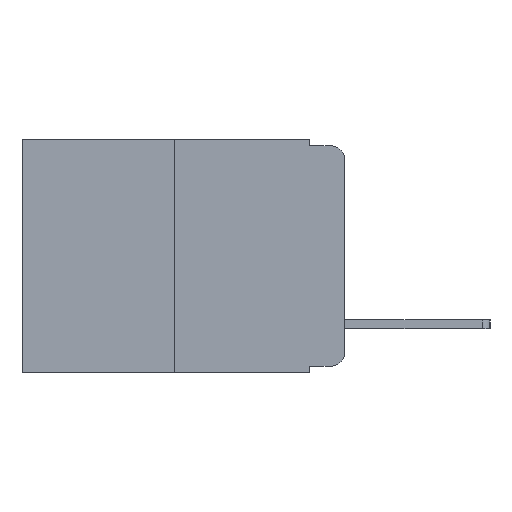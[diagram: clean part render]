
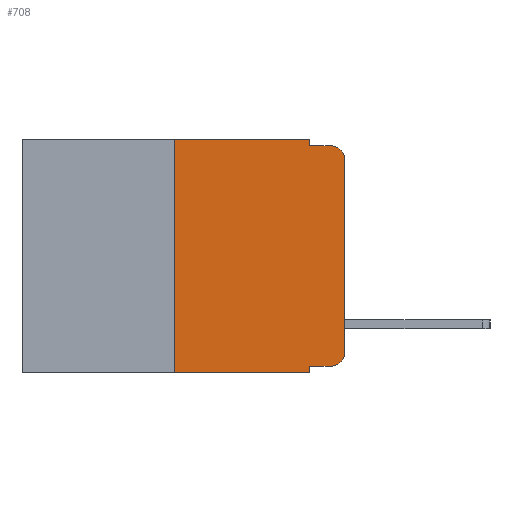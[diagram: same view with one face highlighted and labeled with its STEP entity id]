
A CAD part, left-side view. The second image highlights one B-rep face of the part: STEP entity #708.
In plain terms, the highlighted planar face has unit normal (-1, 0, 0).
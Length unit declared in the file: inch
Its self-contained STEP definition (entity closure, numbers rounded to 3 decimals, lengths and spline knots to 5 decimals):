
#176 = CARTESIAN_POINT ( 'NONE',  ( 0., 0., -0.313 ) ) ;
#244 = CARTESIAN_POINT ( 'NONE',  ( 0., 0.051, -0.343 ) ) ;
#591 = DIRECTION ( 'NONE',  ( 1., 0., 0. ) ) ;
#621 = EDGE_LOOP ( 'NONE', ( #4690, #4538, #4570, #3474, #10437, #2712, #2686, #2624, #2608, #2598 ) ) ;
#708 = ADVANCED_FACE ( 'NONE', ( #4076 ), #6364, .F. ) ;
#753 = EDGE_CURVE ( 'NONE', #4466, #1044, #3719, .T. ) ;
#900 = EDGE_CURVE ( 'NONE', #9452, #3844, #11891, .T. ) ;
#1044 = VERTEX_POINT ( 'NONE', #11967 ) ;
#1226 = LINE ( 'NONE', #13006, #11706 ) ;
#1295 = CARTESIAN_POINT ( 'NONE',  ( 0., 0.02, -0.313 ) ) ;
#1497 = CARTESIAN_POINT ( 'NONE',  ( 0., 0.02, -0.333 ) ) ;
#1512 = VECTOR ( 'NONE', #2199, 39.37008 ) ;
#1514 = DIRECTION ( 'NONE',  ( 0., -1., 0. ) ) ;
#1570 = DIRECTION ( 'NONE',  ( 0., 0., -1. ) ) ;
#1658 = EDGE_CURVE ( 'NONE', #8271, #4466, #1226, .T. ) ;
#1700 = EDGE_CURVE ( 'NONE', #1044, #4318, #10461, .T. ) ;
#1795 = EDGE_CURVE ( 'NONE', #4318, #2188, #11257, .T. ) ;
#1800 = EDGE_CURVE ( 'NONE', #4982, #2188, #8947, .T. ) ;
#1835 = EDGE_CURVE ( 'NONE', #9452, #11655, #2755, .T. ) ;
#1955 = EDGE_CURVE ( 'NONE', #11603, #4982, #11092, .T. ) ;
#2188 = VERTEX_POINT ( 'NONE', #4158 ) ;
#2197 = AXIS2_PLACEMENT_3D ( 'NONE', #13150, #591, #1570 ) ;
#2199 = DIRECTION ( 'NONE',  ( 0., -1., 0. ) ) ;
#2549 = DIRECTION ( 'NONE',  ( 0., 0., -1. ) ) ;
#2598 = ORIENTED_EDGE ( 'NONE', *, *, #9502, .T. ) ;
#2608 = ORIENTED_EDGE ( 'NONE', *, *, #900, .T. ) ;
#2624 = ORIENTED_EDGE ( 'NONE', *, *, #1835, .F. ) ;
#2686 = ORIENTED_EDGE ( 'NONE', *, *, #10506, .T. ) ;
#2712 = ORIENTED_EDGE ( 'NONE', *, *, #1658, .F. ) ;
#2755 = LINE ( 'NONE', #12177, #3091 ) ;
#2957 = CIRCLE ( 'NONE', #13082, 0.02 ) ;
#3091 = VECTOR ( 'NONE', #13109, 39.37008 ) ;
#3105 = DIRECTION ( 'NONE',  ( 0., 0., -1. ) ) ;
#3474 = ORIENTED_EDGE ( 'NONE', *, *, #1700, .F. ) ;
#3578 = VECTOR ( 'NONE', #9287, 39.37008 ) ;
#3719 = LINE ( 'NONE', #8532, #8023 ) ;
#3844 = VERTEX_POINT ( 'NONE', #1497 ) ;
#4076 = FACE_OUTER_BOUND ( 'NONE', #621, .T. ) ;
#4158 = CARTESIAN_POINT ( 'NONE',  ( 0., 0.02, -0.01 ) ) ;
#4306 = VECTOR ( 'NONE', #1514, 39.37008 ) ;
#4318 = VERTEX_POINT ( 'NONE', #10363 ) ;
#4466 = VERTEX_POINT ( 'NONE', #10489 ) ;
#4538 = ORIENTED_EDGE ( 'NONE', *, *, #1800, .T. ) ;
#4570 = ORIENTED_EDGE ( 'NONE', *, *, #1795, .F. ) ;
#4690 = ORIENTED_EDGE ( 'NONE', *, *, #1955, .T. ) ;
#4833 = CARTESIAN_POINT ( 'NONE',  ( 0., 0., 0. ) ) ;
#4837 = CARTESIAN_POINT ( 'NONE',  ( 0., 0.473, -0.343 ) ) ;
#4982 = VERTEX_POINT ( 'NONE', #11196 ) ;
#5270 = AXIS2_PLACEMENT_3D ( 'NONE', #8631, #13480, #13471 ) ;
#5436 = VECTOR ( 'NONE', #3105, 39.37008 ) ;
#5617 = CARTESIAN_POINT ( 'NONE',  ( 0., 0.051, -0.333 ) ) ;
#5806 = CARTESIAN_POINT ( 'NONE',  ( 0., 0.25, -0.343 ) ) ;
#6315 = DIRECTION ( 'NONE',  ( 0., -1., 0. ) ) ;
#6364 = PLANE ( 'NONE',  #2197 ) ;
#8023 = VECTOR ( 'NONE', #10622, 39.37008 ) ;
#8271 = VERTEX_POINT ( 'NONE', #5806 ) ;
#8474 = DIRECTION ( 'NONE',  ( -1., 0., 0. ) ) ;
#8489 = CARTESIAN_POINT ( 'NONE',  ( 0., 0.051, -0.01 ) ) ;
#8532 = CARTESIAN_POINT ( 'NONE',  ( 0., 0.473, 0. ) ) ;
#8628 = VECTOR ( 'NONE', #6315, 39.37008 ) ;
#8631 = CARTESIAN_POINT ( 'NONE',  ( 0., 0.02, -0.03 ) ) ;
#8947 = CIRCLE ( 'NONE', #5270, 0.02 ) ;
#9287 = DIRECTION ( 'NONE',  ( 0., 0., 1. ) ) ;
#9335 = CARTESIAN_POINT ( 'NONE',  ( 0., 0.051, -0.333 ) ) ;
#9452 = VERTEX_POINT ( 'NONE', #5617 ) ;
#9502 = EDGE_CURVE ( 'NONE', #3844, #11603, #2957, .T. ) ;
#10363 = CARTESIAN_POINT ( 'NONE',  ( 0., 0.051, -0.01 ) ) ;
#10437 = ORIENTED_EDGE ( 'NONE', *, *, #753, .F. ) ;
#10461 = LINE ( 'NONE', #13172, #5436 ) ;
#10489 = CARTESIAN_POINT ( 'NONE',  ( 0., 0.25, 0. ) ) ;
#10506 = EDGE_CURVE ( 'NONE', #8271, #11655, #12001, .T. ) ;
#10622 = DIRECTION ( 'NONE',  ( 0., -1., 0. ) ) ;
#10641 = DIRECTION ( 'NONE',  ( 0., 0., 1. ) ) ;
#11092 = LINE ( 'NONE', #4833, #3578 ) ;
#11196 = CARTESIAN_POINT ( 'NONE',  ( 0., 0., -0.03 ) ) ;
#11257 = LINE ( 'NONE', #8489, #8628 ) ;
#11603 = VERTEX_POINT ( 'NONE', #176 ) ;
#11655 = VERTEX_POINT ( 'NONE', #244 ) ;
#11706 = VECTOR ( 'NONE', #10641, 39.37008 ) ;
#11891 = LINE ( 'NONE', #9335, #1512 ) ;
#11967 = CARTESIAN_POINT ( 'NONE',  ( 0., 0.051, 0. ) ) ;
#12001 = LINE ( 'NONE', #4837, #4306 ) ;
#12177 = CARTESIAN_POINT ( 'NONE',  ( 0., 0.051, 0. ) ) ;
#13006 = CARTESIAN_POINT ( 'NONE',  ( 0., 0.25, 0. ) ) ;
#13082 = AXIS2_PLACEMENT_3D ( 'NONE', #1295, #8474, #2549 ) ;
#13109 = DIRECTION ( 'NONE',  ( 0., 0., -1. ) ) ;
#13150 = CARTESIAN_POINT ( 'NONE',  ( 0., 0.473, 0. ) ) ;
#13172 = CARTESIAN_POINT ( 'NONE',  ( 0., 0.051, 0. ) ) ;
#13471 = DIRECTION ( 'NONE',  ( 0., 0., -1. ) ) ;
#13480 = DIRECTION ( 'NONE',  ( -1., 0., 0. ) ) ;
